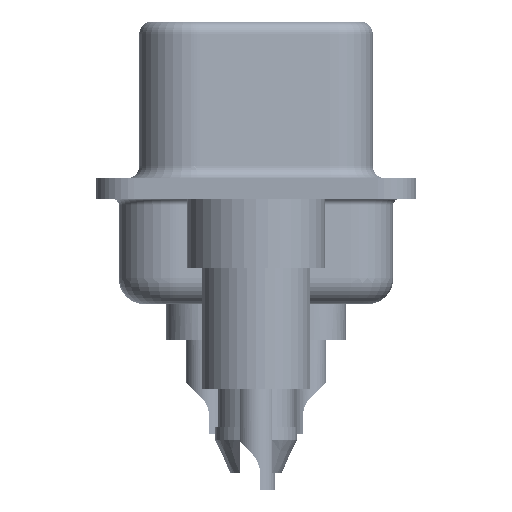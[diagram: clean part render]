
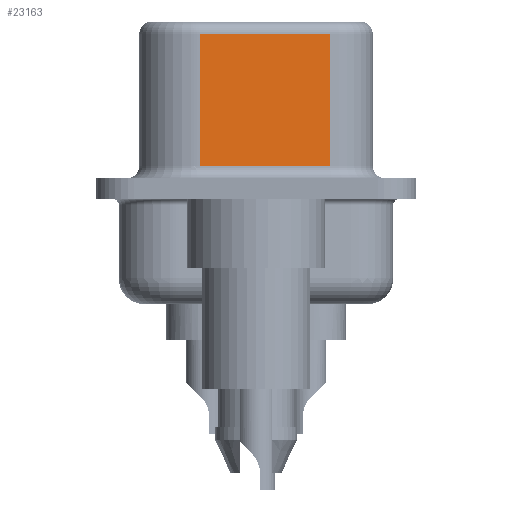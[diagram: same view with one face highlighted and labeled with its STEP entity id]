
A CAD part, left-side view. The second image highlights one B-rep face of the part: STEP entity #23163.
In plain terms, the highlighted planar face has unit normal (-0.985, -0.174, 0).
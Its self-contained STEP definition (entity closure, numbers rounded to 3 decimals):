
#225 = LINE ( 'NONE', #31969, #20261 ) ;
#1247 = CARTESIAN_POINT ( 'NONE',  ( 4.58, -2.897, 0.9 ) ) ;
#2219 = DIRECTION ( 'NONE',  ( 0., 0., -1. ) ) ;
#2310 = DIRECTION ( 'NONE',  ( -0.174, 0.985, 0. ) ) ;
#3748 = ORIENTED_EDGE ( 'NONE', *, *, #13043, .T. ) ;
#3784 = VECTOR ( 'NONE', #13184, 1000. ) ;
#3998 = EDGE_CURVE ( 'NONE', #32935, #23490, #225, .T. ) ;
#4423 = VECTOR ( 'NONE', #2219, 1000. ) ;
#4525 = EDGE_CURVE ( 'NONE', #32935, #27155, #22692, .T. ) ;
#5448 = ORIENTED_EDGE ( 'NONE', *, *, #4525, .T. ) ;
#5521 = ORIENTED_EDGE ( 'NONE', *, *, #3998, .F. ) ;
#8884 = VECTOR ( 'NONE', #2310, 1000. ) ;
#9036 = PLANE ( 'NONE',  #20978 ) ;
#9929 = FACE_OUTER_BOUND ( 'NONE', #17835, .T. ) ;
#10135 = ORIENTED_EDGE ( 'NONE', *, *, #17831, .T. ) ;
#10956 = CARTESIAN_POINT ( 'NONE',  ( 3.68, 2.203, 6.02 ) ) ;
#11449 = LINE ( 'NONE', #12689, #4423 ) ;
#11661 = DIRECTION ( 'NONE',  ( -0.174, 0.985, 0. ) ) ;
#12689 = CARTESIAN_POINT ( 'NONE',  ( 3.68, 2.203, 6.52 ) ) ;
#13043 = EDGE_CURVE ( 'NONE', #14327, #23490, #23764, .T. ) ;
#13184 = DIRECTION ( 'NONE',  ( 0.174, -0.985, 0. ) ) ;
#14114 = CARTESIAN_POINT ( 'NONE',  ( 4.58, -2.897, 6.52 ) ) ;
#14327 = VERTEX_POINT ( 'NONE', #26435 ) ;
#14621 = DIRECTION ( 'NONE',  ( 0., 0., -1. ) ) ;
#15271 = CARTESIAN_POINT ( 'NONE',  ( 4.58, -2.897, 6.02 ) ) ;
#15629 = CARTESIAN_POINT ( 'NONE',  ( 4.58, -2.897, 6.02 ) ) ;
#17831 = EDGE_CURVE ( 'NONE', #27155, #14327, #11449, .T. ) ;
#17835 = EDGE_LOOP ( 'NONE', ( #5521, #5448, #10135, #3748 ) ) ;
#20261 = VECTOR ( 'NONE', #14621, 1000. ) ;
#20978 = AXIS2_PLACEMENT_3D ( 'NONE', #14114, #27103, #11661 ) ;
#21028 = CARTESIAN_POINT ( 'NONE',  ( 4.58, -2.897, 0.9 ) ) ;
#22692 = LINE ( 'NONE', #15271, #8884 ) ;
#23163 = ADVANCED_FACE ( 'NONE', ( #9929 ), #9036, .F. ) ;
#23490 = VERTEX_POINT ( 'NONE', #1247 ) ;
#23764 = LINE ( 'NONE', #21028, #3784 ) ;
#26435 = CARTESIAN_POINT ( 'NONE',  ( 3.68, 2.203, 0.9 ) ) ;
#27103 = DIRECTION ( 'NONE',  ( 0.985, 0.174, 0. ) ) ;
#27155 = VERTEX_POINT ( 'NONE', #10956 ) ;
#31969 = CARTESIAN_POINT ( 'NONE',  ( 4.58, -2.897, 6.52 ) ) ;
#32935 = VERTEX_POINT ( 'NONE', #15629 ) ;
